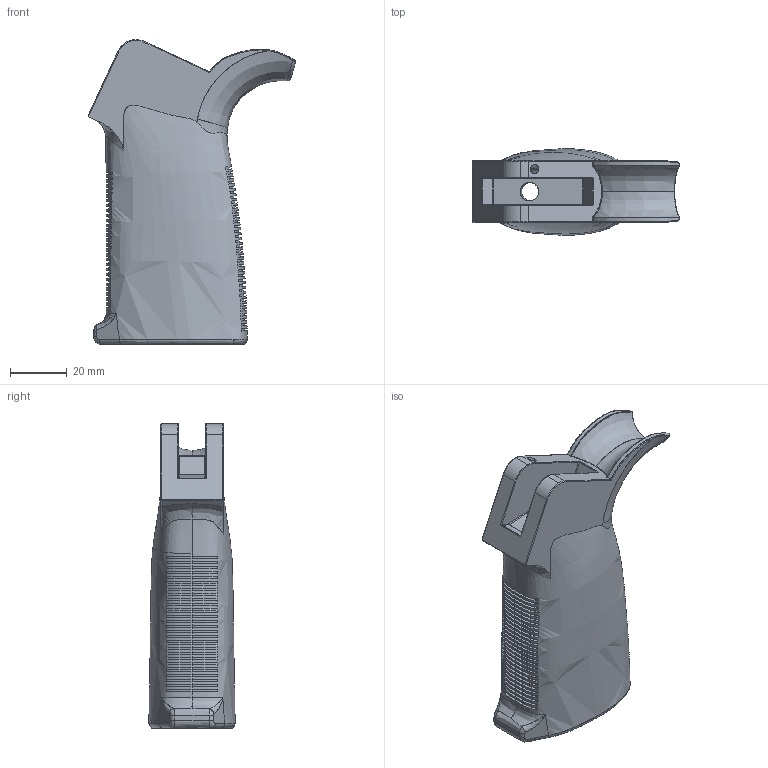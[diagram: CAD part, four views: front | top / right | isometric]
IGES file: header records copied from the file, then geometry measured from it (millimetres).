
Start section: SolidWorks IGES file using analytic representation for surfaces
Global section: file name: GRIP.IGS; native system: SolidWorks 2015; preprocessor: SolidWorks 2015; author: AK0490; date: 150901.183003; units: millimetre
Bounding box: 73.05 x 30.32 x 107.06 mm (x, y, z)
Surface area: 26541.6 mm2 (no closed solid volume)
Topology: 0 solids, 0 shells, 529 faces, 9630 edges, 9625 vertices
Faces by surface type: bspline 475, revolution 54
